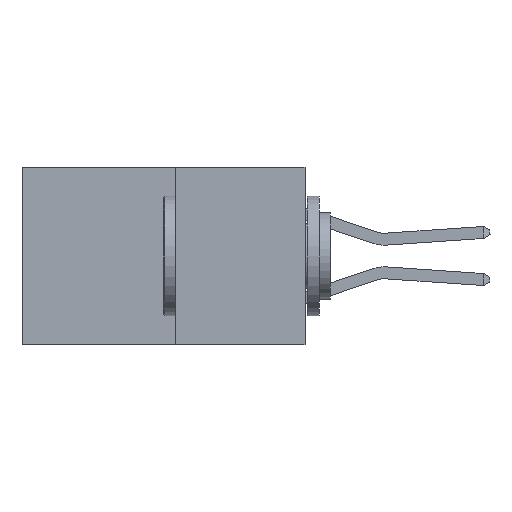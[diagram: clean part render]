
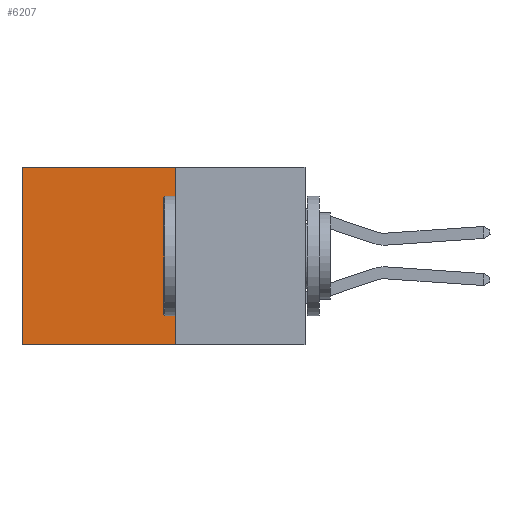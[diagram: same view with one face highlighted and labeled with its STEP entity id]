
A CAD part, left-side view. The second image highlights one B-rep face of the part: STEP entity #6207.
In plain terms, the highlighted planar face has unit normal (-1, 0, 0).
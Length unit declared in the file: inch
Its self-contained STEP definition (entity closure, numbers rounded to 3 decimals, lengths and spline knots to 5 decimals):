
#39 = LINE ( 'NONE', #7766, #2525 ) ;
#223 = AXIS2_PLACEMENT_3D ( 'NONE', #6263, #6419, #6773 ) ;
#255 = CARTESIAN_POINT ( 'NONE',  ( 0.277, 0.27, -0.37 ) ) ;
#264 = CARTESIAN_POINT ( 'NONE',  ( 0.277, 0.27, -0.37 ) ) ;
#611 = EDGE_LOOP ( 'NONE', ( #2622, #2806, #3027, #3188 ) ) ;
#1549 = EDGE_CURVE ( 'NONE', #9136, #5928, #11013, .T. ) ;
#1843 = CARTESIAN_POINT ( 'NONE',  ( 0.277, 0.27, -0.37 ) ) ;
#1960 = DIRECTION ( 'NONE',  ( 0., 0., -1. ) ) ;
#2418 = EDGE_CURVE ( 'NONE', #7757, #5928, #39, .T. ) ;
#2525 = VECTOR ( 'NONE', #7914, 39.37008 ) ;
#2622 = ORIENTED_EDGE ( 'NONE', *, *, #2418, .T. ) ;
#2783 = LINE ( 'NONE', #3171, #5101 ) ;
#2806 = ORIENTED_EDGE ( 'NONE', *, *, #1549, .F. ) ;
#3027 = ORIENTED_EDGE ( 'NONE', *, *, #5697, .F. ) ;
#3171 = CARTESIAN_POINT ( 'NONE',  ( 0.277, 0.27, 0. ) ) ;
#3188 = ORIENTED_EDGE ( 'NONE', *, *, #10111, .T. ) ;
#3784 = VECTOR ( 'NONE', #1960, 39.37008 ) ;
#3863 = CARTESIAN_POINT ( 'NONE',  ( 0.277, 0.27, 0. ) ) ;
#4043 = DIRECTION ( 'NONE',  ( 0., 1., 0. ) ) ;
#5101 = VECTOR ( 'NONE', #4043, 39.37008 ) ;
#5605 = VERTEX_POINT ( 'NONE', #3863 ) ;
#5631 = DIRECTION ( 'NONE',  ( 0., 1., 0. ) ) ;
#5697 = EDGE_CURVE ( 'NONE', #5605, #9136, #8288, .T. ) ;
#5928 = VERTEX_POINT ( 'NONE', #5971 ) ;
#5971 = CARTESIAN_POINT ( 'NONE',  ( 0.277, 0.59, -0.37 ) ) ;
#6207 = ADVANCED_FACE ( 'NONE', ( #7977 ), #6426, .F. ) ;
#6260 = CARTESIAN_POINT ( 'NONE',  ( 0.277, 0.59, 0. ) ) ;
#6263 = CARTESIAN_POINT ( 'NONE',  ( 0.277, 0.27, -0.37 ) ) ;
#6419 = DIRECTION ( 'NONE',  ( 1., 0., 0. ) ) ;
#6426 = PLANE ( 'NONE',  #223 ) ;
#6773 = DIRECTION ( 'NONE',  ( 0., 0., -1. ) ) ;
#7757 = VERTEX_POINT ( 'NONE', #6260 ) ;
#7766 = CARTESIAN_POINT ( 'NONE',  ( 0.277, 0.59, -0.37 ) ) ;
#7914 = DIRECTION ( 'NONE',  ( 0., 0., -1. ) ) ;
#7977 = FACE_OUTER_BOUND ( 'NONE', #611, .T. ) ;
#8288 = LINE ( 'NONE', #1843, #3784 ) ;
#9136 = VERTEX_POINT ( 'NONE', #255 ) ;
#10111 = EDGE_CURVE ( 'NONE', #5605, #7757, #2783, .T. ) ;
#10759 = VECTOR ( 'NONE', #5631, 39.37008 ) ;
#11013 = LINE ( 'NONE', #264, #10759 ) ;
